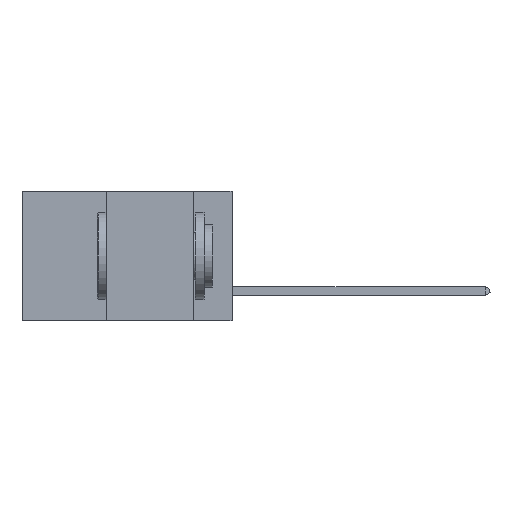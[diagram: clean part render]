
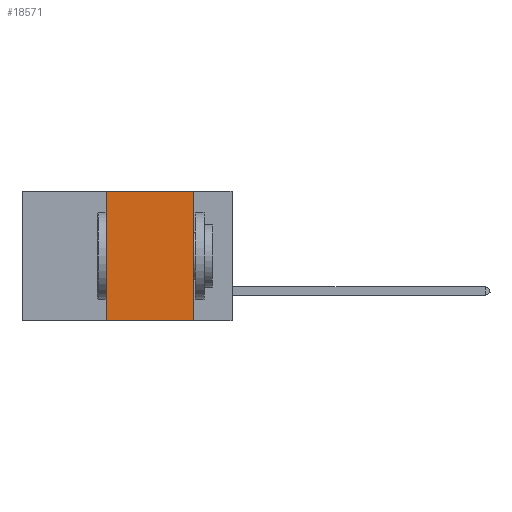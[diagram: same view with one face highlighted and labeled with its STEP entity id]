
A CAD part, left-side view. The second image highlights one B-rep face of the part: STEP entity #18571.
In plain terms, the highlighted planar face has unit normal (-1, 0, 0).
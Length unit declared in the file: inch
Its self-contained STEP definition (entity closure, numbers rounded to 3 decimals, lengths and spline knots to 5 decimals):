
#1833 = LINE ( 'NONE', #9640, #6693 ) ;
#2013 = PLANE ( 'NONE',  #8198 ) ;
#4271 = LINE ( 'NONE', #6176, #13464 ) ;
#4696 = EDGE_CURVE ( 'NONE', #18953, #20719, #4271, .T. ) ;
#5001 = ORIENTED_EDGE ( 'NONE', *, *, #21704, .F. ) ;
#5341 = ORIENTED_EDGE ( 'NONE', *, *, #18001, .F. ) ;
#6051 = ORIENTED_EDGE ( 'NONE', *, *, #4696, .F. ) ;
#6176 = CARTESIAN_POINT ( 'NONE',  ( 0., 0.6, 0. ) ) ;
#6693 = VECTOR ( 'NONE', #16701, 39.37008 ) ;
#6842 = DIRECTION ( 'NONE',  ( 1., 0., 0. ) ) ;
#8198 = AXIS2_PLACEMENT_3D ( 'NONE', #8711, #6842, #15705 ) ;
#8711 = CARTESIAN_POINT ( 'NONE',  ( 0., 0.6, 0. ) ) ;
#8781 = EDGE_LOOP ( 'NONE', ( #5001, #6051, #5341, #10904 ) ) ;
#9486 = VECTOR ( 'NONE', #20317, 39.37008 ) ;
#9628 = FACE_OUTER_BOUND ( 'NONE', #8781, .T. ) ;
#9640 = CARTESIAN_POINT ( 'NONE',  ( 0., 0.36, 0. ) ) ;
#9714 = DIRECTION ( 'NONE',  ( 0., -1., 0. ) ) ;
#10161 = CARTESIAN_POINT ( 'NONE',  ( 0., 0.11, 0. ) ) ;
#10904 = ORIENTED_EDGE ( 'NONE', *, *, #16204, .T. ) ;
#12359 = VERTEX_POINT ( 'NONE', #16398 ) ;
#12726 = CARTESIAN_POINT ( 'NONE',  ( 0., 0.6, -0.37 ) ) ;
#13464 = VECTOR ( 'NONE', #9714, 39.37008 ) ;
#14098 = LINE ( 'NONE', #10161, #9486 ) ;
#14528 = DIRECTION ( 'NONE',  ( 0., -1., 0. ) ) ;
#15294 = CARTESIAN_POINT ( 'NONE',  ( 0., 0.36, 0. ) ) ;
#15705 = DIRECTION ( 'NONE',  ( 0., 0., -1. ) ) ;
#15845 = CARTESIAN_POINT ( 'NONE',  ( 0., 0.36, -0.37 ) ) ;
#16204 = EDGE_CURVE ( 'NONE', #17157, #12359, #21034, .T. ) ;
#16398 = CARTESIAN_POINT ( 'NONE',  ( 0., 0.11, -0.37 ) ) ;
#16701 = DIRECTION ( 'NONE',  ( 0., 0., 1. ) ) ;
#17157 = VERTEX_POINT ( 'NONE', #15845 ) ;
#18001 = EDGE_CURVE ( 'NONE', #17157, #18953, #1833, .T. ) ;
#18571 = ADVANCED_FACE ( 'NONE', ( #9628 ), #2013, .F. ) ;
#18953 = VERTEX_POINT ( 'NONE', #15294 ) ;
#19401 = VECTOR ( 'NONE', #14528, 39.37008 ) ;
#19899 = CARTESIAN_POINT ( 'NONE',  ( 0., 0.11, 0. ) ) ;
#20317 = DIRECTION ( 'NONE',  ( 0., 0., -1. ) ) ;
#20719 = VERTEX_POINT ( 'NONE', #19899 ) ;
#21034 = LINE ( 'NONE', #12726, #19401 ) ;
#21704 = EDGE_CURVE ( 'NONE', #20719, #12359, #14098, .T. ) ;
